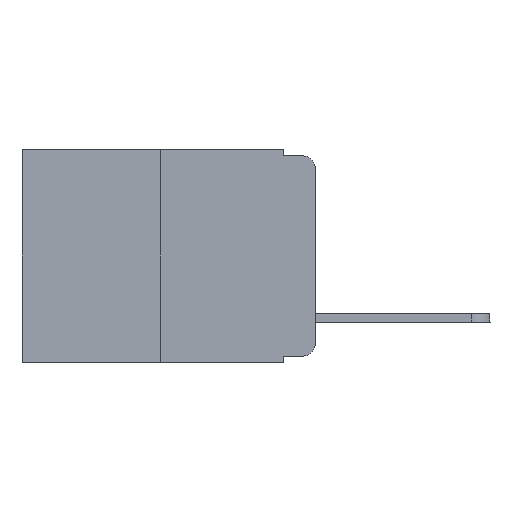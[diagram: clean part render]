
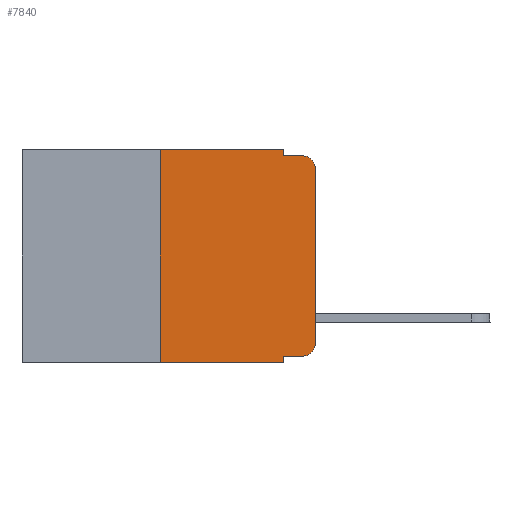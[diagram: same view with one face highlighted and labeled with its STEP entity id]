
A CAD part, left-side view. The second image highlights one B-rep face of the part: STEP entity #7840.
In plain terms, the highlighted planar face has unit normal (-1, 0, 0).
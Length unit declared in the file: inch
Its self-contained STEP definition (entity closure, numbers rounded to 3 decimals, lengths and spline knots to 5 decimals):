
#72 = EDGE_CURVE ( 'NONE', #9031, #11169, #10137, .T. ) ;
#114 = DIRECTION ( 'NONE',  ( 0., 0., -1. ) ) ;
#430 = EDGE_CURVE ( 'NONE', #14788, #12037, #21502, .T. ) ;
#817 = CARTESIAN_POINT ( 'NONE',  ( 0., 0.051, 0. ) ) ;
#1854 = EDGE_CURVE ( 'NONE', #9092, #16182, #14480, .T. ) ;
#2169 = DIRECTION ( 'NONE',  ( 0., -1., 0. ) ) ;
#2439 = DIRECTION ( 'NONE',  ( 0., 0., 1. ) ) ;
#2516 = CARTESIAN_POINT ( 'NONE',  ( 0., 0.25, -0.343 ) ) ;
#2771 = LINE ( 'NONE', #7516, #7510 ) ;
#2842 = DIRECTION ( 'NONE',  ( 0., 0., -1. ) ) ;
#3548 = VECTOR ( 'NONE', #8084, 39.37008 ) ;
#4092 = CARTESIAN_POINT ( 'NONE',  ( 0., 0.051, -0.333 ) ) ;
#4537 = CARTESIAN_POINT ( 'NONE',  ( 0., 0.473, 0. ) ) ;
#4795 = VERTEX_POINT ( 'NONE', #20879 ) ;
#5249 = ORIENTED_EDGE ( 'NONE', *, *, #25425, .F. ) ;
#5376 = VECTOR ( 'NONE', #11417, 39.37008 ) ;
#7012 = EDGE_CURVE ( 'NONE', #14938, #9031, #24618, .T. ) ;
#7213 = VERTEX_POINT ( 'NONE', #14197 ) ;
#7510 = VECTOR ( 'NONE', #15184, 39.37008 ) ;
#7516 = CARTESIAN_POINT ( 'NONE',  ( 0., 0., 0. ) ) ;
#7810 = EDGE_CURVE ( 'NONE', #10456, #7213, #24894, .T. ) ;
#7840 = ADVANCED_FACE ( 'NONE', ( #8780 ), #18761, .F. ) ;
#7864 = CARTESIAN_POINT ( 'NONE',  ( 0., 0.051, -0.01 ) ) ;
#8084 = DIRECTION ( 'NONE',  ( 0., -1., 0. ) ) ;
#8232 = CARTESIAN_POINT ( 'NONE',  ( 0., 0.02, -0.313 ) ) ;
#8302 = ORIENTED_EDGE ( 'NONE', *, *, #72, .T. ) ;
#8356 = LINE ( 'NONE', #9729, #17855 ) ;
#8423 = CARTESIAN_POINT ( 'NONE',  ( 0., 0.25, 0. ) ) ;
#8533 = EDGE_CURVE ( 'NONE', #11169, #9092, #2771, .T. ) ;
#8780 = FACE_OUTER_BOUND ( 'NONE', #16818, .T. ) ;
#9031 = VERTEX_POINT ( 'NONE', #24905 ) ;
#9092 = VERTEX_POINT ( 'NONE', #15221 ) ;
#9298 = ORIENTED_EDGE ( 'NONE', *, *, #16211, .F. ) ;
#9729 = CARTESIAN_POINT ( 'NONE',  ( 0., 0.473, 0. ) ) ;
#10080 = ORIENTED_EDGE ( 'NONE', *, *, #7810, .F. ) ;
#10137 = CIRCLE ( 'NONE', #17678, 0.02 ) ;
#10171 = DIRECTION ( 'NONE',  ( -1., 0., 0. ) ) ;
#10274 = DIRECTION ( 'NONE',  ( 1., 0., 0. ) ) ;
#10456 = VERTEX_POINT ( 'NONE', #2516 ) ;
#10548 = DIRECTION ( 'NONE',  ( 0., 0., -1. ) ) ;
#11169 = VERTEX_POINT ( 'NONE', #15881 ) ;
#11417 = DIRECTION ( 'NONE',  ( 0., 0., -1. ) ) ;
#11582 = CARTESIAN_POINT ( 'NONE',  ( 0., 0.051, 0. ) ) ;
#11623 = ORIENTED_EDGE ( 'NONE', *, *, #15750, .T. ) ;
#11643 = DIRECTION ( 'NONE',  ( 0., 0., -1. ) ) ;
#11681 = CARTESIAN_POINT ( 'NONE',  ( 0., 0.051, 0. ) ) ;
#12037 = VERTEX_POINT ( 'NONE', #7864 ) ;
#12444 = ORIENTED_EDGE ( 'NONE', *, *, #7012, .T. ) ;
#12731 = LINE ( 'NONE', #20172, #3548 ) ;
#12964 = DIRECTION ( 'NONE',  ( 0., -1., 0. ) ) ;
#13250 = ORIENTED_EDGE ( 'NONE', *, *, #8533, .T. ) ;
#13673 = CARTESIAN_POINT ( 'NONE',  ( 0., 0.02, -0.03 ) ) ;
#13754 = ORIENTED_EDGE ( 'NONE', *, *, #18519, .F. ) ;
#14170 = VECTOR ( 'NONE', #2439, 39.37008 ) ;
#14197 = CARTESIAN_POINT ( 'NONE',  ( 0., 0.25, 0. ) ) ;
#14220 = VECTOR ( 'NONE', #2169, 39.37008 ) ;
#14345 = LINE ( 'NONE', #817, #14989 ) ;
#14480 = CIRCLE ( 'NONE', #15508, 0.02 ) ;
#14578 = VECTOR ( 'NONE', #12964, 39.37008 ) ;
#14788 = VERTEX_POINT ( 'NONE', #11681 ) ;
#14938 = VERTEX_POINT ( 'NONE', #15979 ) ;
#14989 = VECTOR ( 'NONE', #2842, 39.37008 ) ;
#15184 = DIRECTION ( 'NONE',  ( 0., 0., 1. ) ) ;
#15221 = CARTESIAN_POINT ( 'NONE',  ( 0., 0., -0.03 ) ) ;
#15508 = AXIS2_PLACEMENT_3D ( 'NONE', #13673, #15846, #11643 ) ;
#15750 = EDGE_CURVE ( 'NONE', #10456, #4795, #21834, .T. ) ;
#15845 = ORIENTED_EDGE ( 'NONE', *, *, #430, .F. ) ;
#15846 = DIRECTION ( 'NONE',  ( -1., 0., 0. ) ) ;
#15881 = CARTESIAN_POINT ( 'NONE',  ( 0., 0., -0.313 ) ) ;
#15979 = CARTESIAN_POINT ( 'NONE',  ( 0., 0.051, -0.333 ) ) ;
#16182 = VERTEX_POINT ( 'NONE', #20223 ) ;
#16211 = EDGE_CURVE ( 'NONE', #12037, #16182, #12731, .T. ) ;
#16818 = EDGE_LOOP ( 'NONE', ( #13250, #22884, #9298, #15845, #13754, #10080, #11623, #5249, #12444, #8302 ) ) ;
#17678 = AXIS2_PLACEMENT_3D ( 'NONE', #8232, #10171, #114 ) ;
#17807 = AXIS2_PLACEMENT_3D ( 'NONE', #4537, #10274, #10548 ) ;
#17855 = VECTOR ( 'NONE', #23950, 39.37008 ) ;
#18519 = EDGE_CURVE ( 'NONE', #7213, #14788, #8356, .T. ) ;
#18761 = PLANE ( 'NONE',  #17807 ) ;
#20172 = CARTESIAN_POINT ( 'NONE',  ( 0., 0.051, -0.01 ) ) ;
#20223 = CARTESIAN_POINT ( 'NONE',  ( 0., 0.02, -0.01 ) ) ;
#20879 = CARTESIAN_POINT ( 'NONE',  ( 0., 0.051, -0.343 ) ) ;
#20961 = CARTESIAN_POINT ( 'NONE',  ( 0., 0.473, -0.343 ) ) ;
#21502 = LINE ( 'NONE', #11582, #5376 ) ;
#21834 = LINE ( 'NONE', #20961, #14578 ) ;
#22884 = ORIENTED_EDGE ( 'NONE', *, *, #1854, .T. ) ;
#23950 = DIRECTION ( 'NONE',  ( 0., -1., 0. ) ) ;
#24618 = LINE ( 'NONE', #4092, #14220 ) ;
#24894 = LINE ( 'NONE', #8423, #14170 ) ;
#24905 = CARTESIAN_POINT ( 'NONE',  ( 0., 0.02, -0.333 ) ) ;
#25425 = EDGE_CURVE ( 'NONE', #14938, #4795, #14345, .T. ) ;
